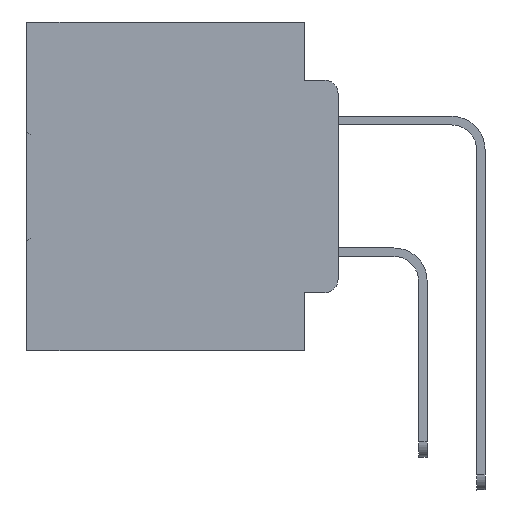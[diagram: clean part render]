
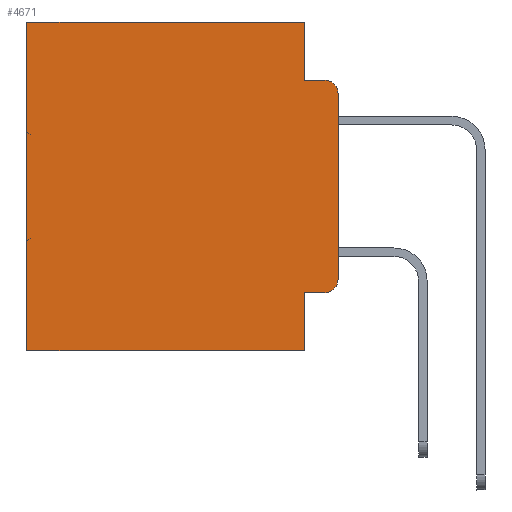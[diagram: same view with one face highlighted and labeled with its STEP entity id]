
A CAD part, left-side view. The second image highlights one B-rep face of the part: STEP entity #4671.
In plain terms, the highlighted planar face has unit normal (-1, 0, 0).
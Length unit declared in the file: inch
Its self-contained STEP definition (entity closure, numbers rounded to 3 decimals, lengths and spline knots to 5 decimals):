
#10 = ORIENTED_EDGE ( 'NONE', *, *, #14753, .F. ) ;
#1194 = VECTOR ( 'NONE', #23690, 39.37008 ) ;
#1254 = CARTESIAN_POINT ( 'NONE',  ( 0.298, 0.051, -0.5 ) ) ;
#1983 = CARTESIAN_POINT ( 'NONE',  ( 0.298, 0.02, -0.0885 ) ) ;
#2035 = DIRECTION ( 'NONE',  ( 0., 0., -1. ) ) ;
#2466 = PLANE ( 'NONE',  #21898 ) ;
#2860 = LINE ( 'NONE', #26311, #31401 ) ;
#3025 = VECTOR ( 'NONE', #2035, 39.37008 ) ;
#3430 = CARTESIAN_POINT ( 'NONE',  ( 0.298, 0., 0. ) ) ;
#3526 = EDGE_CURVE ( 'NONE', #9595, #34444, #26522, .T. ) ;
#3807 = VECTOR ( 'NONE', #17063, 39.37008 ) ;
#4671 = ADVANCED_FACE ( 'NONE', ( #11055 ), #2466, .F. ) ;
#4715 = LINE ( 'NONE', #30702, #3807 ) ;
#4998 = CIRCLE ( 'NONE', #15000, 0.02 ) ;
#5471 = EDGE_CURVE ( 'NONE', #9595, #18495, #8856, .T. ) ;
#5867 = VERTEX_POINT ( 'NONE', #20797 ) ;
#6635 = EDGE_LOOP ( 'NONE', ( #7795, #25834, #10, #27276, #23320, #33352, #33581, #6986, #23256, #33520 ) ) ;
#6986 = ORIENTED_EDGE ( 'NONE', *, *, #5471, .F. ) ;
#7224 = VERTEX_POINT ( 'NONE', #1983 ) ;
#7233 = DIRECTION ( 'NONE',  ( -1., 0., 0. ) ) ;
#7795 = ORIENTED_EDGE ( 'NONE', *, *, #29457, .F. ) ;
#7935 = CARTESIAN_POINT ( 'NONE',  ( 0.298, 0., -0.1085 ) ) ;
#8152 = CARTESIAN_POINT ( 'NONE',  ( 0.298, 0.473, 0. ) ) ;
#8669 = CARTESIAN_POINT ( 'NONE',  ( 0.298, 0.473, 0. ) ) ;
#8856 = LINE ( 'NONE', #9753, #1194 ) ;
#8890 = CARTESIAN_POINT ( 'NONE',  ( 0.298, 0., 0. ) ) ;
#8996 = DIRECTION ( 'NONE',  ( 1., 0., 0. ) ) ;
#9595 = VERTEX_POINT ( 'NONE', #20947 ) ;
#9753 = CARTESIAN_POINT ( 'NONE',  ( 0.298, 0.051, 0. ) ) ;
#9987 = VERTEX_POINT ( 'NONE', #33672 ) ;
#10593 = LINE ( 'NONE', #29640, #3025 ) ;
#10603 = CARTESIAN_POINT ( 'NONE',  ( 0.298, 0.02, -0.3915 ) ) ;
#11055 = FACE_OUTER_BOUND ( 'NONE', #6635, .T. ) ;
#11119 = EDGE_CURVE ( 'NONE', #11638, #12838, #19172, .T. ) ;
#11638 = VERTEX_POINT ( 'NONE', #8152 ) ;
#11858 = DIRECTION ( 'NONE',  ( 0., 0., -1. ) ) ;
#12789 = DIRECTION ( 'NONE',  ( 0., -1., 0. ) ) ;
#12838 = VERTEX_POINT ( 'NONE', #27707 ) ;
#12914 = EDGE_CURVE ( 'NONE', #5867, #18897, #4715, .T. ) ;
#13293 = DIRECTION ( 'NONE',  ( 0., 0., -1. ) ) ;
#13376 = EDGE_CURVE ( 'NONE', #18495, #12838, #2860, .T. ) ;
#13874 = CARTESIAN_POINT ( 'NONE',  ( 0.298, 0.02, -0.4115 ) ) ;
#14753 = EDGE_CURVE ( 'NONE', #18897, #7224, #29579, .T. ) ;
#15000 = AXIS2_PLACEMENT_3D ( 'NONE', #10603, #29734, #13293 ) ;
#17063 = DIRECTION ( 'NONE',  ( 0., 0., -1. ) ) ;
#17076 = VECTOR ( 'NONE', #25395, 39.37008 ) ;
#18341 = VECTOR ( 'NONE', #33285, 39.37008 ) ;
#18363 = VECTOR ( 'NONE', #22286, 39.37008 ) ;
#18495 = VERTEX_POINT ( 'NONE', #1254 ) ;
#18897 = VERTEX_POINT ( 'NONE', #33619 ) ;
#19172 = LINE ( 'NONE', #8669, #18341 ) ;
#19174 = VERTEX_POINT ( 'NONE', #7935 ) ;
#20277 = EDGE_CURVE ( 'NONE', #19174, #7224, #31949, .T. ) ;
#20797 = CARTESIAN_POINT ( 'NONE',  ( 0.298, 0.051, 0. ) ) ;
#20947 = CARTESIAN_POINT ( 'NONE',  ( 0.298, 0.051, -0.4115 ) ) ;
#21898 = AXIS2_PLACEMENT_3D ( 'NONE', #3430, #8996, #11858 ) ;
#22286 = DIRECTION ( 'NONE',  ( 0., -1., 0. ) ) ;
#22332 = VECTOR ( 'NONE', #12789, 39.37008 ) ;
#23256 = ORIENTED_EDGE ( 'NONE', *, *, #3526, .T. ) ;
#23320 = ORIENTED_EDGE ( 'NONE', *, *, #28562, .T. ) ;
#23673 = CARTESIAN_POINT ( 'NONE',  ( 0.298, 0.02, -0.1085 ) ) ;
#23677 = DIRECTION ( 'NONE',  ( 0., 1., 0. ) ) ;
#23690 = DIRECTION ( 'NONE',  ( 0., 0., -1. ) ) ;
#25395 = DIRECTION ( 'NONE',  ( 0., 1., 0. ) ) ;
#25834 = ORIENTED_EDGE ( 'NONE', *, *, #20277, .T. ) ;
#26311 = CARTESIAN_POINT ( 'NONE',  ( 0.298, 0., -0.5 ) ) ;
#26426 = DIRECTION ( 'NONE',  ( 0., 0., -1. ) ) ;
#26522 = LINE ( 'NONE', #34029, #18363 ) ;
#27276 = ORIENTED_EDGE ( 'NONE', *, *, #12914, .F. ) ;
#27707 = CARTESIAN_POINT ( 'NONE',  ( 0.298, 0.473, -0.5 ) ) ;
#27993 = AXIS2_PLACEMENT_3D ( 'NONE', #23673, #7233, #26426 ) ;
#28562 = EDGE_CURVE ( 'NONE', #5867, #11638, #31615, .T. ) ;
#29212 = CARTESIAN_POINT ( 'NONE',  ( 0.298, 0.051, -0.0885 ) ) ;
#29457 = EDGE_CURVE ( 'NONE', #19174, #9987, #10593, .T. ) ;
#29579 = LINE ( 'NONE', #29212, #22332 ) ;
#29640 = CARTESIAN_POINT ( 'NONE',  ( 0.298, 0., 0. ) ) ;
#29734 = DIRECTION ( 'NONE',  ( -1., 0., 0. ) ) ;
#30702 = CARTESIAN_POINT ( 'NONE',  ( 0.298, 0.051, 0. ) ) ;
#31401 = VECTOR ( 'NONE', #23677, 39.37008 ) ;
#31615 = LINE ( 'NONE', #8890, #17076 ) ;
#31949 = CIRCLE ( 'NONE', #27993, 0.02 ) ;
#33285 = DIRECTION ( 'NONE',  ( 0., 0., -1. ) ) ;
#33352 = ORIENTED_EDGE ( 'NONE', *, *, #11119, .T. ) ;
#33520 = ORIENTED_EDGE ( 'NONE', *, *, #33744, .T. ) ;
#33581 = ORIENTED_EDGE ( 'NONE', *, *, #13376, .F. ) ;
#33619 = CARTESIAN_POINT ( 'NONE',  ( 0.298, 0.051, -0.0885 ) ) ;
#33672 = CARTESIAN_POINT ( 'NONE',  ( 0.298, 0., -0.3915 ) ) ;
#33744 = EDGE_CURVE ( 'NONE', #34444, #9987, #4998, .T. ) ;
#34029 = CARTESIAN_POINT ( 'NONE',  ( 0.298, 0.051, -0.4115 ) ) ;
#34444 = VERTEX_POINT ( 'NONE', #13874 ) ;
